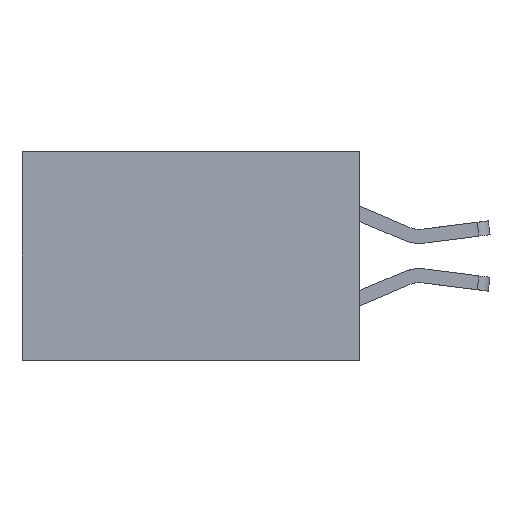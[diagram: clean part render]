
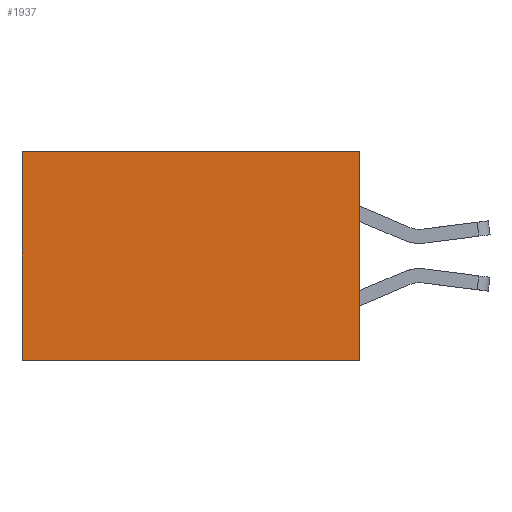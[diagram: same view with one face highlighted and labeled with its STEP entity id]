
A CAD part, left-side view. The second image highlights one B-rep face of the part: STEP entity #1937.
In plain terms, the highlighted planar face has unit normal (-1, 0, 0).
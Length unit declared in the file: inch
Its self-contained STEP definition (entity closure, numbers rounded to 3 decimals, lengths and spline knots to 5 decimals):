
#333 = VERTEX_POINT ( 'NONE', #5717 ) ;
#433 = VECTOR ( 'NONE', #8363, 39.37008 ) ;
#468 = DIRECTION ( 'NONE',  ( 0., 0., -1. ) ) ;
#1150 = VECTOR ( 'NONE', #3525, 39.37008 ) ;
#1597 = EDGE_CURVE ( 'NONE', #3679, #9099, #5506, .T. ) ;
#1603 = CARTESIAN_POINT ( 'NONE',  ( 0.2875, 0.6, 0. ) ) ;
#1716 = AXIS2_PLACEMENT_3D ( 'NONE', #4390, #7241, #4924 ) ;
#1793 = ORIENTED_EDGE ( 'NONE', *, *, #6197, .T. ) ;
#1937 = ADVANCED_FACE ( 'NONE', ( #9384 ), #4702, .F. ) ;
#1996 = LINE ( 'NONE', #3714, #6010 ) ;
#2900 = LINE ( 'NONE', #3619, #433 ) ;
#3525 = DIRECTION ( 'NONE',  ( 0., 1., 0. ) ) ;
#3619 = CARTESIAN_POINT ( 'NONE',  ( 0.2875, 0.6, 0. ) ) ;
#3642 = EDGE_LOOP ( 'NONE', ( #1793, #8474, #9987, #9028 ) ) ;
#3679 = VERTEX_POINT ( 'NONE', #8592 ) ;
#3714 = CARTESIAN_POINT ( 'NONE',  ( 0.2875, 0., 0. ) ) ;
#4261 = VECTOR ( 'NONE', #5880, 39.37008 ) ;
#4390 = CARTESIAN_POINT ( 'NONE',  ( 0.2875, 0., 0. ) ) ;
#4702 = PLANE ( 'NONE',  #1716 ) ;
#4924 = DIRECTION ( 'NONE',  ( 0., 0., -1. ) ) ;
#5065 = CARTESIAN_POINT ( 'NONE',  ( 0.2875, 0., -0.37 ) ) ;
#5506 = LINE ( 'NONE', #9849, #1150 ) ;
#5717 = CARTESIAN_POINT ( 'NONE',  ( 0.2875, 0., -0.37 ) ) ;
#5880 = DIRECTION ( 'NONE',  ( 0., 1., 0. ) ) ;
#6010 = VECTOR ( 'NONE', #468, 39.37008 ) ;
#6197 = EDGE_CURVE ( 'NONE', #9099, #7540, #2900, .T. ) ;
#6549 = EDGE_CURVE ( 'NONE', #3679, #333, #1996, .T. ) ;
#7241 = DIRECTION ( 'NONE',  ( 1., 0., 0. ) ) ;
#7540 = VERTEX_POINT ( 'NONE', #7672 ) ;
#7672 = CARTESIAN_POINT ( 'NONE',  ( 0.2875, 0.6, -0.37 ) ) ;
#8363 = DIRECTION ( 'NONE',  ( 0., 0., -1. ) ) ;
#8474 = ORIENTED_EDGE ( 'NONE', *, *, #8659, .F. ) ;
#8592 = CARTESIAN_POINT ( 'NONE',  ( 0.2875, 0., 0. ) ) ;
#8659 = EDGE_CURVE ( 'NONE', #333, #7540, #8689, .T. ) ;
#8689 = LINE ( 'NONE', #5065, #4261 ) ;
#9028 = ORIENTED_EDGE ( 'NONE', *, *, #1597, .T. ) ;
#9099 = VERTEX_POINT ( 'NONE', #1603 ) ;
#9384 = FACE_OUTER_BOUND ( 'NONE', #3642, .T. ) ;
#9849 = CARTESIAN_POINT ( 'NONE',  ( 0.2875, 0., 0. ) ) ;
#9987 = ORIENTED_EDGE ( 'NONE', *, *, #6549, .F. ) ;
